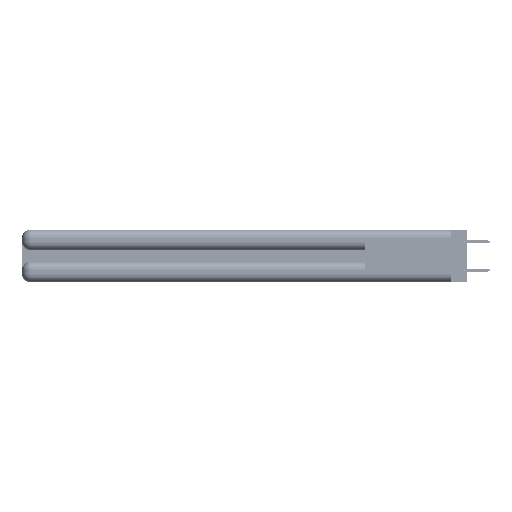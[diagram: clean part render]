
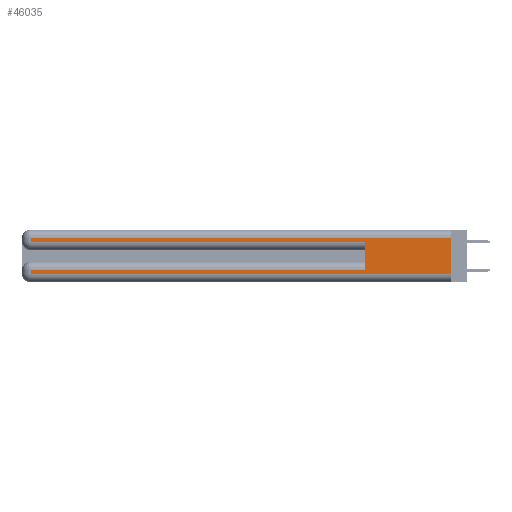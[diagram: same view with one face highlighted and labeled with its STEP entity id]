
A CAD part, left-side view. The second image highlights one B-rep face of the part: STEP entity #46035.
In plain terms, the highlighted planar face has unit normal (-1, 0, 0).
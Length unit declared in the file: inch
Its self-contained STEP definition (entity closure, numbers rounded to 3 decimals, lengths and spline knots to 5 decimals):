
#483 = EDGE_CURVE ( 'NONE', #49416, #53993, #51926, .T. ) ;
#2932 = LINE ( 'NONE', #47485, #15727 ) ;
#2945 = LINE ( 'NONE', #3174, #17708 ) ;
#3174 = CARTESIAN_POINT ( 'NONE',  ( 0., 0., 0.06 ) ) ;
#3690 = VECTOR ( 'NONE', #53979, 39.37008 ) ;
#4416 = CARTESIAN_POINT ( 'NONE',  ( 0., 0.6, 0.085 ) ) ;
#5601 = VERTEX_POINT ( 'NONE', #7475 ) ;
#6137 = VECTOR ( 'NONE', #53490, 39.37008 ) ;
#6351 = ORIENTED_EDGE ( 'NONE', *, *, #17724, .T. ) ;
#7475 = CARTESIAN_POINT ( 'NONE',  ( 0., 0., 0.31 ) ) ;
#7704 = ORIENTED_EDGE ( 'NONE', *, *, #8607, .T. ) ;
#8607 = EDGE_CURVE ( 'NONE', #32773, #16683, #35358, .T. ) ;
#9136 = PLANE ( 'NONE',  #33360 ) ;
#12566 = EDGE_CURVE ( 'NONE', #49416, #24421, #2932, .T. ) ;
#13593 = EDGE_CURVE ( 'NONE', #5601, #42784, #48034, .T. ) ;
#13905 = DIRECTION ( 'NONE',  ( 0., 1., 0. ) ) ;
#14429 = LINE ( 'NONE', #19719, #3690 ) ;
#14442 = CARTESIAN_POINT ( 'NONE',  ( 0., 2.94, 0.06 ) ) ;
#15130 = LINE ( 'NONE', #36181, #37410 ) ;
#15172 = CARTESIAN_POINT ( 'NONE',  ( 0., 0., 0.285 ) ) ;
#15396 = ORIENTED_EDGE ( 'NONE', *, *, #13593, .F. ) ;
#15727 = VECTOR ( 'NONE', #17049, 39.37008 ) ;
#16575 = CARTESIAN_POINT ( 'NONE',  ( 0., 2.94, 0.285 ) ) ;
#16683 = VERTEX_POINT ( 'NONE', #16575 ) ;
#17049 = DIRECTION ( 'NONE',  ( 0., 0., 1. ) ) ;
#17147 = CARTESIAN_POINT ( 'NONE',  ( 0., 0.6, 0.285 ) ) ;
#17708 = VECTOR ( 'NONE', #29353, 39.37008 ) ;
#17724 = EDGE_CURVE ( 'NONE', #16683, #24421, #31329, .T. ) ;
#18314 = CARTESIAN_POINT ( 'NONE',  ( 0., 0., 0.37 ) ) ;
#18750 = VECTOR ( 'NONE', #13905, 39.37008 ) ;
#19719 = CARTESIAN_POINT ( 'NONE',  ( 0., 0., 0.31 ) ) ;
#21583 = ORIENTED_EDGE ( 'NONE', *, *, #43925, .T. ) ;
#21869 = ORIENTED_EDGE ( 'NONE', *, *, #12566, .F. ) ;
#22547 = ORIENTED_EDGE ( 'NONE', *, *, #38610, .T. ) ;
#24208 = DIRECTION ( 'NONE',  ( 0., -1., 0. ) ) ;
#24421 = VERTEX_POINT ( 'NONE', #17147 ) ;
#27728 = CARTESIAN_POINT ( 'NONE',  ( 0., 2.94, 0.37 ) ) ;
#27813 = EDGE_LOOP ( 'NONE', ( #15396, #42778, #7704, #6351, #21869, #42743, #21583, #22547 ) ) ;
#29298 = VERTEX_POINT ( 'NONE', #14442 ) ;
#29353 = DIRECTION ( 'NONE',  ( 0., -1., 0. ) ) ;
#31329 = LINE ( 'NONE', #15172, #40748 ) ;
#32773 = VERTEX_POINT ( 'NONE', #48110 ) ;
#33360 = AXIS2_PLACEMENT_3D ( 'NONE', #52205, #52573, #34620 ) ;
#34620 = DIRECTION ( 'NONE',  ( 0., 0., -1. ) ) ;
#35358 = LINE ( 'NONE', #27728, #42765 ) ;
#36136 = CARTESIAN_POINT ( 'NONE',  ( 0., 2.94, 0.085 ) ) ;
#36181 = CARTESIAN_POINT ( 'NONE',  ( 0., 2.94, 0.37 ) ) ;
#37410 = VECTOR ( 'NONE', #44864, 39.37008 ) ;
#38610 = EDGE_CURVE ( 'NONE', #29298, #42784, #2945, .T. ) ;
#40748 = VECTOR ( 'NONE', #24208, 39.37008 ) ;
#42743 = ORIENTED_EDGE ( 'NONE', *, *, #483, .T. ) ;
#42765 = VECTOR ( 'NONE', #44741, 39.37008 ) ;
#42778 = ORIENTED_EDGE ( 'NONE', *, *, #43983, .T. ) ;
#42784 = VERTEX_POINT ( 'NONE', #54842 ) ;
#43925 = EDGE_CURVE ( 'NONE', #53993, #29298, #15130, .T. ) ;
#43983 = EDGE_CURVE ( 'NONE', #5601, #32773, #14429, .T. ) ;
#44296 = CARTESIAN_POINT ( 'NONE',  ( 0., 0., 0.085 ) ) ;
#44741 = DIRECTION ( 'NONE',  ( 0., 0., -1. ) ) ;
#44864 = DIRECTION ( 'NONE',  ( 0., 0., -1. ) ) ;
#46035 = ADVANCED_FACE ( 'NONE', ( #53123 ), #9136, .F. ) ;
#47485 = CARTESIAN_POINT ( 'NONE',  ( 0., 0.6, 0.145 ) ) ;
#48034 = LINE ( 'NONE', #18314, #6137 ) ;
#48110 = CARTESIAN_POINT ( 'NONE',  ( 0., 2.94, 0.31 ) ) ;
#49416 = VERTEX_POINT ( 'NONE', #4416 ) ;
#51926 = LINE ( 'NONE', #44296, #18750 ) ;
#52205 = CARTESIAN_POINT ( 'NONE',  ( 0., 0., 0.37 ) ) ;
#52573 = DIRECTION ( 'NONE',  ( 1., 0., 0. ) ) ;
#53123 = FACE_OUTER_BOUND ( 'NONE', #27813, .T. ) ;
#53490 = DIRECTION ( 'NONE',  ( 0., 0., -1. ) ) ;
#53979 = DIRECTION ( 'NONE',  ( 0., 1., 0. ) ) ;
#53993 = VERTEX_POINT ( 'NONE', #36136 ) ;
#54842 = CARTESIAN_POINT ( 'NONE',  ( 0., 0., 0.06 ) ) ;
